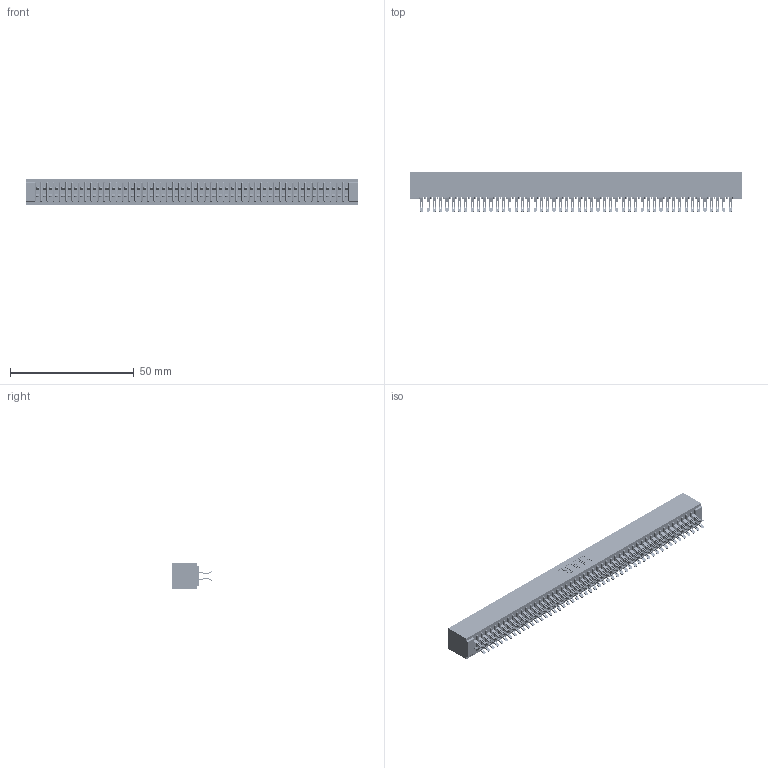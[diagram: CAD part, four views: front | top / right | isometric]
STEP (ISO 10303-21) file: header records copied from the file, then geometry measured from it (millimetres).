
FILE_DESCRIPTION (( 'STEP AP203' ), '1' );
FILE_NAME ('391-100-555-201.STEP', '2018-08-09T19:33:36', ( '' ), ( '' ), 'SwSTEP 2.0', 'SolidWorks 2016', '' );
FILE_SCHEMA (( 'CONFIG_CONTROL_DESIGN' ));
Length unit declared in the file: inch
Products named in the file (3): 341 Part_No Mounting Lugs; 341-292-001_341-292-155; 391-100-555-201
Assembly tree (101 placements, depth 2):
  391-100-555-201
    341 Part_No Mounting Lugs
    341-292-001_341-292-155  x100
Bounding box: 133.99 x 16.31 x 10.16 mm (x, y, z)
Volume: 10264.1 mm3; surface area: 19951 mm2
Topology: 101 solids, 101 shells, 7908 faces, 23642 edges, 15390 vertices
Faces by surface type: plane 4264, cylinder 3444, sphere 102, torus 98
Entity records: 59637 total; most frequent: CARTESIAN_POINT 9928, ORIENTED_EDGE 9856, DIRECTION 9618, EDGE_CURVE 4928, VECTOR 3978, LINE 3978, VERTEX_POINT 3114, AXIS2_PLACEMENT_3D 2820
